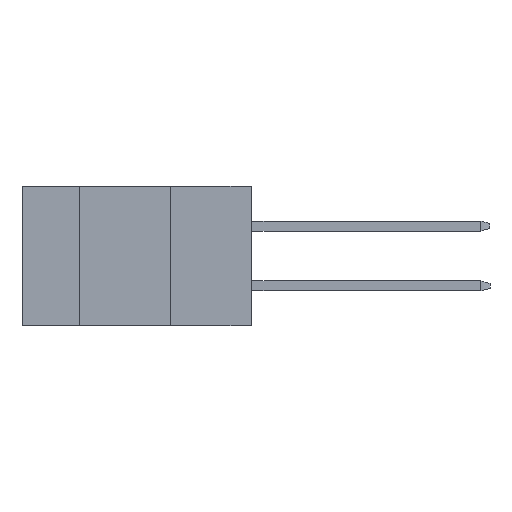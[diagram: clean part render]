
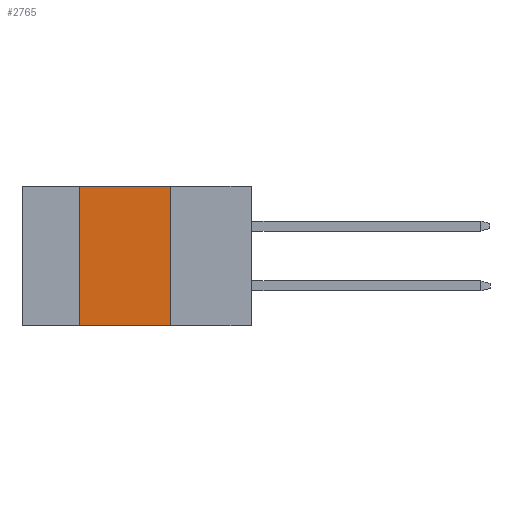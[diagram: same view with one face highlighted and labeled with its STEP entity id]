
A CAD part, left-side view. The second image highlights one B-rep face of the part: STEP entity #2765.
In plain terms, the highlighted planar face has unit normal (-1, 0, 0).
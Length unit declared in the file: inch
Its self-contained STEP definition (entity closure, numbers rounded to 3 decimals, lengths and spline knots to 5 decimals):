
#75 = CARTESIAN_POINT ( 'NONE',  ( 0., 0.54, -0.437 ) ) ;
#417 = LINE ( 'NONE', #9123, #15253 ) ;
#835 = CARTESIAN_POINT ( 'NONE',  ( 0., 0.254, 0. ) ) ;
#1990 = CARTESIAN_POINT ( 'NONE',  ( 0., 0.72, 0. ) ) ;
#2765 = ADVANCED_FACE ( 'NONE', ( #14975 ), #6273, .F. ) ;
#3845 = VECTOR ( 'NONE', #5477, 39.37008 ) ;
#4041 = EDGE_CURVE ( 'NONE', #8284, #15408, #10180, .T. ) ;
#4309 = LINE ( 'NONE', #10441, #13071 ) ;
#4345 = EDGE_CURVE ( 'NONE', #16270, #8284, #16652, .T. ) ;
#4867 = VECTOR ( 'NONE', #15212, 39.37008 ) ;
#5477 = DIRECTION ( 'NONE',  ( 0., -1., 0. ) ) ;
#6273 = PLANE ( 'NONE',  #16154 ) ;
#6283 = EDGE_CURVE ( 'NONE', #15408, #12634, #4309, .T. ) ;
#7578 = DIRECTION ( 'NONE',  ( 0., -1., 0. ) ) ;
#8284 = VERTEX_POINT ( 'NONE', #16480 ) ;
#8683 = EDGE_CURVE ( 'NONE', #16270, #12634, #417, .T. ) ;
#9123 = CARTESIAN_POINT ( 'NONE',  ( 0., 0.72, -0.437 ) ) ;
#9404 = CARTESIAN_POINT ( 'NONE',  ( 0., 0.54, -0.437 ) ) ;
#10180 = LINE ( 'NONE', #18764, #3845 ) ;
#10199 = CARTESIAN_POINT ( 'NONE',  ( 0., 0.254, -0.437 ) ) ;
#10441 = CARTESIAN_POINT ( 'NONE',  ( 0., 0.254, -0.437 ) ) ;
#11990 = ORIENTED_EDGE ( 'NONE', *, *, #8683, .T. ) ;
#12634 = VERTEX_POINT ( 'NONE', #10199 ) ;
#13071 = VECTOR ( 'NONE', #18836, 39.37008 ) ;
#13542 = EDGE_LOOP ( 'NONE', ( #15523, #14407, #14001, #11990 ) ) ;
#14001 = ORIENTED_EDGE ( 'NONE', *, *, #4345, .F. ) ;
#14407 = ORIENTED_EDGE ( 'NONE', *, *, #4041, .F. ) ;
#14700 = DIRECTION ( 'NONE',  ( 0., 0., -1. ) ) ;
#14975 = FACE_OUTER_BOUND ( 'NONE', #13542, .T. ) ;
#15212 = DIRECTION ( 'NONE',  ( 0., 0., 1. ) ) ;
#15253 = VECTOR ( 'NONE', #7578, 39.37008 ) ;
#15408 = VERTEX_POINT ( 'NONE', #835 ) ;
#15523 = ORIENTED_EDGE ( 'NONE', *, *, #6283, .F. ) ;
#16154 = AXIS2_PLACEMENT_3D ( 'NONE', #1990, #17852, #14700 ) ;
#16270 = VERTEX_POINT ( 'NONE', #75 ) ;
#16480 = CARTESIAN_POINT ( 'NONE',  ( 0., 0.54, 0. ) ) ;
#16652 = LINE ( 'NONE', #9404, #4867 ) ;
#17852 = DIRECTION ( 'NONE',  ( 1., 0., 0. ) ) ;
#18764 = CARTESIAN_POINT ( 'NONE',  ( 0., 0.72, 0. ) ) ;
#18836 = DIRECTION ( 'NONE',  ( 0., 0., -1. ) ) ;
